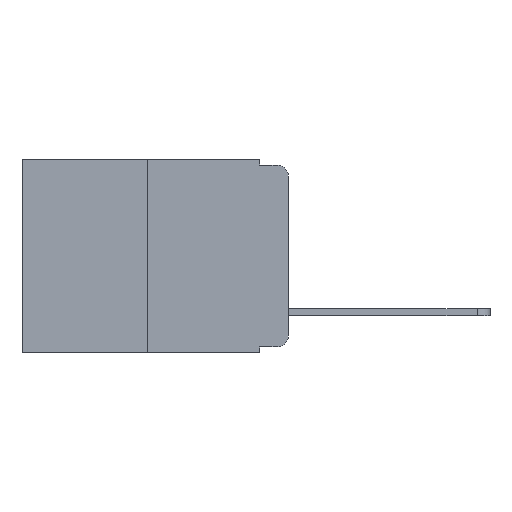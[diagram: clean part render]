
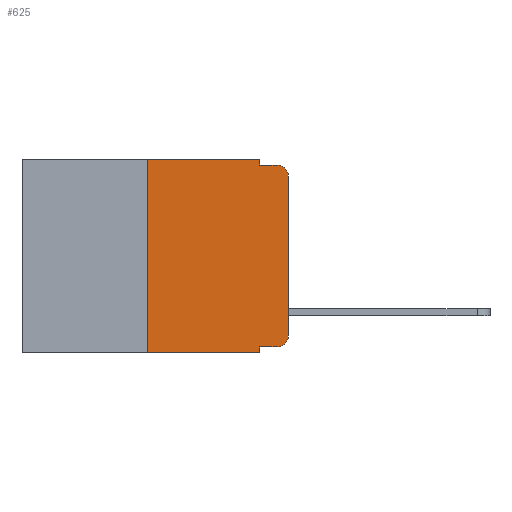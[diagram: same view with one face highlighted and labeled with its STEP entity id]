
A CAD part, left-side view. The second image highlights one B-rep face of the part: STEP entity #625.
In plain terms, the highlighted planar face has unit normal (-1, 0, 0).
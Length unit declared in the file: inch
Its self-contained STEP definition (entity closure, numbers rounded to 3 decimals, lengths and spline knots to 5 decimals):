
#109 = ORIENTED_EDGE ( 'NONE', *, *, #8427, .F. ) ;
#537 = ORIENTED_EDGE ( 'NONE', *, *, #6506, .F. ) ;
#625 = ADVANCED_FACE ( 'NONE', ( #1677 ), #12291, .F. ) ;
#638 = DIRECTION ( 'NONE',  ( 0., 0., 1. ) ) ;
#647 = CARTESIAN_POINT ( 'NONE',  ( 0., 0.051, -0.01 ) ) ;
#1102 = ORIENTED_EDGE ( 'NONE', *, *, #10313, .T. ) ;
#1121 = ORIENTED_EDGE ( 'NONE', *, *, #3379, .T. ) ;
#1677 = FACE_OUTER_BOUND ( 'NONE', #2218, .T. ) ;
#1713 = ORIENTED_EDGE ( 'NONE', *, *, #5728, .F. ) ;
#1896 = VERTEX_POINT ( 'NONE', #10983 ) ;
#1916 = VERTEX_POINT ( 'NONE', #6848 ) ;
#1975 = VERTEX_POINT ( 'NONE', #10470 ) ;
#2218 = EDGE_LOOP ( 'NONE', ( #5389, #5069, #1713, #3126, #537, #109, #8282, #8344, #1102, #1121 ) ) ;
#2634 = VECTOR ( 'NONE', #7504, 39.37008 ) ;
#2646 = DIRECTION ( 'NONE',  ( 0., 0., -1. ) ) ;
#3064 = VERTEX_POINT ( 'NONE', #8367 ) ;
#3126 = ORIENTED_EDGE ( 'NONE', *, *, #6419, .F. ) ;
#3148 = VERTEX_POINT ( 'NONE', #12475 ) ;
#3299 = CARTESIAN_POINT ( 'NONE',  ( 0., 0., -0.03 ) ) ;
#3379 = EDGE_CURVE ( 'NONE', #3064, #1916, #4896, .T. ) ;
#3658 = EDGE_CURVE ( 'NONE', #1916, #10285, #11292, .T. ) ;
#3856 = LINE ( 'NONE', #5834, #8607 ) ;
#4030 = LINE ( 'NONE', #647, #12105 ) ;
#4474 = VERTEX_POINT ( 'NONE', #12284 ) ;
#4665 = DIRECTION ( 'NONE',  ( 0., 0., -1. ) ) ;
#4896 = CIRCLE ( 'NONE', #12138, 0.02 ) ;
#4928 = AXIS2_PLACEMENT_3D ( 'NONE', #12427, #8895, #11956 ) ;
#5059 = EDGE_CURVE ( 'NONE', #10285, #7475, #9804, .T. ) ;
#5069 = ORIENTED_EDGE ( 'NONE', *, *, #5059, .T. ) ;
#5200 = VERTEX_POINT ( 'NONE', #11882 ) ;
#5389 = ORIENTED_EDGE ( 'NONE', *, *, #3658, .T. ) ;
#5475 = LINE ( 'NONE', #6485, #2634 ) ;
#5723 = CARTESIAN_POINT ( 'NONE',  ( 0., 0.25, 0. ) ) ;
#5728 = EDGE_CURVE ( 'NONE', #10232, #7475, #4030, .T. ) ;
#5766 = VECTOR ( 'NONE', #6309, 39.37008 ) ;
#5834 = CARTESIAN_POINT ( 'NONE',  ( 0., 0.473, -0.343 ) ) ;
#5971 = EDGE_CURVE ( 'NONE', #1896, #3148, #3856, .T. ) ;
#5997 = CARTESIAN_POINT ( 'NONE',  ( 0., 0., 0. ) ) ;
#6258 = CARTESIAN_POINT ( 'NONE',  ( 0., 0.473, 0. ) ) ;
#6309 = DIRECTION ( 'NONE',  ( 0., -1., 0. ) ) ;
#6411 = LINE ( 'NONE', #6258, #5766 ) ;
#6419 = EDGE_CURVE ( 'NONE', #5200, #10232, #9918, .T. ) ;
#6485 = CARTESIAN_POINT ( 'NONE',  ( 0., 0.051, -0.333 ) ) ;
#6506 = EDGE_CURVE ( 'NONE', #1975, #5200, #6411, .T. ) ;
#6848 = CARTESIAN_POINT ( 'NONE',  ( 0., 0., -0.313 ) ) ;
#7475 = VERTEX_POINT ( 'NONE', #10836 ) ;
#7504 = DIRECTION ( 'NONE',  ( 0., -1., 0. ) ) ;
#7618 = DIRECTION ( 'NONE',  ( 0., 0., -1. ) ) ;
#7691 = VECTOR ( 'NONE', #7618, 39.37008 ) ;
#7763 = DIRECTION ( 'NONE',  ( 0., 0., 1. ) ) ;
#7969 = DIRECTION ( 'NONE',  ( 0., -1., 0. ) ) ;
#8282 = ORIENTED_EDGE ( 'NONE', *, *, #5971, .T. ) ;
#8344 = ORIENTED_EDGE ( 'NONE', *, *, #9059, .F. ) ;
#8367 = CARTESIAN_POINT ( 'NONE',  ( 0., 0.02, -0.333 ) ) ;
#8404 = LINE ( 'NONE', #5723, #12992 ) ;
#8427 = EDGE_CURVE ( 'NONE', #1896, #1975, #8404, .T. ) ;
#8508 = CARTESIAN_POINT ( 'NONE',  ( 0., 0.051, 0. ) ) ;
#8607 = VECTOR ( 'NONE', #9167, 39.37008 ) ;
#8642 = CARTESIAN_POINT ( 'NONE',  ( 0., 0.051, 0. ) ) ;
#8791 = VECTOR ( 'NONE', #638, 39.37008 ) ;
#8799 = DIRECTION ( 'NONE',  ( -1., 0., 0. ) ) ;
#8895 = DIRECTION ( 'NONE',  ( 1., 0., 0. ) ) ;
#9059 = EDGE_CURVE ( 'NONE', #4474, #3148, #9132, .T. ) ;
#9132 = LINE ( 'NONE', #8642, #11336 ) ;
#9167 = DIRECTION ( 'NONE',  ( 0., -1., 0. ) ) ;
#9280 = CARTESIAN_POINT ( 'NONE',  ( 0., 0.051, -0.01 ) ) ;
#9639 = DIRECTION ( 'NONE',  ( 0., 0., -1. ) ) ;
#9804 = CIRCLE ( 'NONE', #10088, 0.02 ) ;
#9918 = LINE ( 'NONE', #8508, #7691 ) ;
#10088 = AXIS2_PLACEMENT_3D ( 'NONE', #11573, #10205, #9639 ) ;
#10205 = DIRECTION ( 'NONE',  ( -1., 0., 0. ) ) ;
#10232 = VERTEX_POINT ( 'NONE', #9280 ) ;
#10285 = VERTEX_POINT ( 'NONE', #3299 ) ;
#10313 = EDGE_CURVE ( 'NONE', #4474, #3064, #5475, .T. ) ;
#10470 = CARTESIAN_POINT ( 'NONE',  ( 0., 0.25, 0. ) ) ;
#10836 = CARTESIAN_POINT ( 'NONE',  ( 0., 0.02, -0.01 ) ) ;
#10983 = CARTESIAN_POINT ( 'NONE',  ( 0., 0.25, -0.343 ) ) ;
#11292 = LINE ( 'NONE', #5997, #8791 ) ;
#11336 = VECTOR ( 'NONE', #4665, 39.37008 ) ;
#11573 = CARTESIAN_POINT ( 'NONE',  ( 0., 0.02, -0.03 ) ) ;
#11705 = CARTESIAN_POINT ( 'NONE',  ( 0., 0.02, -0.313 ) ) ;
#11882 = CARTESIAN_POINT ( 'NONE',  ( 0., 0.051, 0. ) ) ;
#11956 = DIRECTION ( 'NONE',  ( 0., 0., -1. ) ) ;
#12105 = VECTOR ( 'NONE', #7969, 39.37008 ) ;
#12138 = AXIS2_PLACEMENT_3D ( 'NONE', #11705, #8799, #2646 ) ;
#12284 = CARTESIAN_POINT ( 'NONE',  ( 0., 0.051, -0.333 ) ) ;
#12291 = PLANE ( 'NONE',  #4928 ) ;
#12427 = CARTESIAN_POINT ( 'NONE',  ( 0., 0.473, 0. ) ) ;
#12475 = CARTESIAN_POINT ( 'NONE',  ( 0., 0.051, -0.343 ) ) ;
#12992 = VECTOR ( 'NONE', #7763, 39.37008 ) ;
